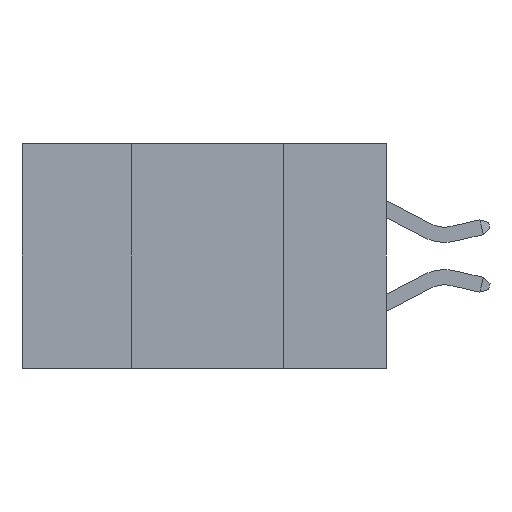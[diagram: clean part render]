
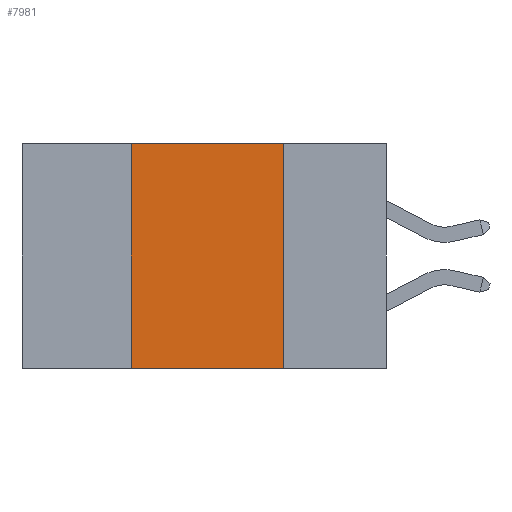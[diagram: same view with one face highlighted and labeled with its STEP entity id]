
A CAD part, left-side view. The second image highlights one B-rep face of the part: STEP entity #7981.
In plain terms, the highlighted planar face has unit normal (-1, 0, 0).
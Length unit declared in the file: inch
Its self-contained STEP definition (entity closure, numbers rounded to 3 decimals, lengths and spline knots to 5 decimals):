
#448 = VERTEX_POINT ( 'NONE', #6294 ) ;
#864 = DIRECTION ( 'NONE',  ( 0., 0., 1. ) ) ;
#1027 = EDGE_CURVE ( 'NONE', #448, #5404, #7492, .T. ) ;
#1394 = CARTESIAN_POINT ( 'NONE',  ( 0., 0.42, -0.37 ) ) ;
#1709 = VECTOR ( 'NONE', #7035, 39.37008 ) ;
#1986 = EDGE_CURVE ( 'NONE', #13472, #7093, #15292, .T. ) ;
#2320 = DIRECTION ( 'NONE',  ( 0., 0., -1. ) ) ;
#2351 = DIRECTION ( 'NONE',  ( 1., 0., 0. ) ) ;
#3486 = DIRECTION ( 'NONE',  ( 0., -1., 0. ) ) ;
#3764 = FACE_OUTER_BOUND ( 'NONE', #16435, .T. ) ;
#4325 = CARTESIAN_POINT ( 'NONE',  ( 0., 0.17, -0.37 ) ) ;
#5343 = PLANE ( 'NONE',  #15636 ) ;
#5404 = VERTEX_POINT ( 'NONE', #4325 ) ;
#5454 = CARTESIAN_POINT ( 'NONE',  ( 0., 0.6, 0. ) ) ;
#5545 = ORIENTED_EDGE ( 'NONE', *, *, #8124, .T. ) ;
#6162 = VECTOR ( 'NONE', #3486, 39.37008 ) ;
#6294 = CARTESIAN_POINT ( 'NONE',  ( 0., 0.17, 0. ) ) ;
#7035 = DIRECTION ( 'NONE',  ( 0., -1., 0. ) ) ;
#7093 = VERTEX_POINT ( 'NONE', #8496 ) ;
#7483 = CARTESIAN_POINT ( 'NONE',  ( 0., 0.6, -0.37 ) ) ;
#7492 = LINE ( 'NONE', #11194, #13981 ) ;
#7981 = ADVANCED_FACE ( 'NONE', ( #3764 ), #5343, .F. ) ;
#8124 = EDGE_CURVE ( 'NONE', #13472, #5404, #12125, .T. ) ;
#8450 = VECTOR ( 'NONE', #864, 39.37008 ) ;
#8496 = CARTESIAN_POINT ( 'NONE',  ( 0., 0.42, 0. ) ) ;
#8555 = ORIENTED_EDGE ( 'NONE', *, *, #1027, .F. ) ;
#9442 = ORIENTED_EDGE ( 'NONE', *, *, #1986, .F. ) ;
#9629 = LINE ( 'NONE', #12603, #6162 ) ;
#11194 = CARTESIAN_POINT ( 'NONE',  ( 0., 0.17, -0.37 ) ) ;
#12125 = LINE ( 'NONE', #7483, #1709 ) ;
#12268 = DIRECTION ( 'NONE',  ( 0., 0., -1. ) ) ;
#12603 = CARTESIAN_POINT ( 'NONE',  ( 0., 0.6, 0. ) ) ;
#13068 = CARTESIAN_POINT ( 'NONE',  ( 0., 0.42, -0.37 ) ) ;
#13472 = VERTEX_POINT ( 'NONE', #13068 ) ;
#13981 = VECTOR ( 'NONE', #12268, 39.37008 ) ;
#15292 = LINE ( 'NONE', #1394, #8450 ) ;
#15636 = AXIS2_PLACEMENT_3D ( 'NONE', #5454, #2351, #2320 ) ;
#16253 = ORIENTED_EDGE ( 'NONE', *, *, #16625, .F. ) ;
#16435 = EDGE_LOOP ( 'NONE', ( #8555, #16253, #9442, #5545 ) ) ;
#16625 = EDGE_CURVE ( 'NONE', #7093, #448, #9629, .T. ) ;
